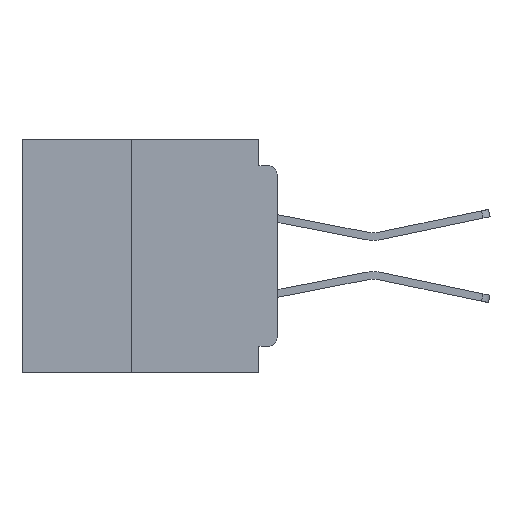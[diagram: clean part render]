
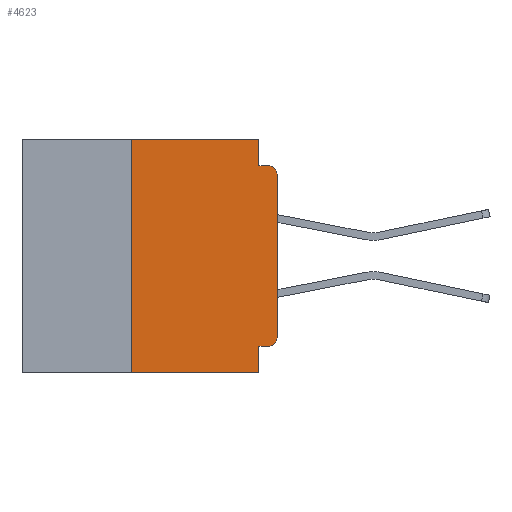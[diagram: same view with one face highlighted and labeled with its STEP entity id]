
A CAD part, left-side view. The second image highlights one B-rep face of the part: STEP entity #4623.
In plain terms, the highlighted planar face has unit normal (-1, 0, 0).
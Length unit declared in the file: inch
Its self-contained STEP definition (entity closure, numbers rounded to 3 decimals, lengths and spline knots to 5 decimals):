
#2740 = AXIS2_PLACEMENT_3D ( 'NONE', #12466, #54005, #53925 ) ;
#3252 = DIRECTION ( 'NONE',  ( 0., -1., 0. ) ) ;
#4163 = EDGE_CURVE ( 'NONE', #45471, #45231, #57447, .T. ) ;
#4395 = LINE ( 'NONE', #33269, #16461 ) ;
#4623 = ADVANCED_FACE ( 'NONE', ( #21454 ), #52763, .F. ) ;
#4956 = DIRECTION ( 'NONE',  ( 0., 0., 1. ) ) ;
#6588 = EDGE_CURVE ( 'NONE', #56029, #7572, #48117, .T. ) ;
#7572 = VERTEX_POINT ( 'NONE', #36489 ) ;
#8348 = DIRECTION ( 'NONE',  ( -1., 0., 0. ) ) ;
#8466 = VERTEX_POINT ( 'NONE', #13797 ) ;
#9559 = ORIENTED_EDGE ( 'NONE', *, *, #12828, .F. ) ;
#11077 = VERTEX_POINT ( 'NONE', #17024 ) ;
#11893 = LINE ( 'NONE', #43286, #58418 ) ;
#12466 = CARTESIAN_POINT ( 'NONE',  ( 0., 0.437, 0. ) ) ;
#12828 = EDGE_CURVE ( 'NONE', #22465, #34806, #11893, .T. ) ;
#13797 = CARTESIAN_POINT ( 'NONE',  ( 0., 0.25, 0. ) ) ;
#14143 = CARTESIAN_POINT ( 'NONE',  ( 0., 0., -0.355 ) ) ;
#14544 = CARTESIAN_POINT ( 'NONE',  ( 0., 0.031, -0.045 ) ) ;
#15021 = ORIENTED_EDGE ( 'NONE', *, *, #6588, .T. ) ;
#15884 = DIRECTION ( 'NONE',  ( -1., 0., 0. ) ) ;
#16260 = DIRECTION ( 'NONE',  ( 0., -1., 0. ) ) ;
#16461 = VECTOR ( 'NONE', #55725, 39.37008 ) ;
#16549 = CARTESIAN_POINT ( 'NONE',  ( 0., 0.015, -0.355 ) ) ;
#16623 = VECTOR ( 'NONE', #16260, 39.37008 ) ;
#17024 = CARTESIAN_POINT ( 'NONE',  ( 0., 0.031, -0.4 ) ) ;
#17712 = EDGE_CURVE ( 'NONE', #42472, #11077, #4395, .T. ) ;
#18859 = ORIENTED_EDGE ( 'NONE', *, *, #36431, .F. ) ;
#21454 = FACE_OUTER_BOUND ( 'NONE', #23707, .T. ) ;
#22059 = EDGE_CURVE ( 'NONE', #34806, #55670, #52582, .T. ) ;
#22465 = VERTEX_POINT ( 'NONE', #33381 ) ;
#23034 = DIRECTION ( 'NONE',  ( 0., 1., 0. ) ) ;
#23264 = ORIENTED_EDGE ( 'NONE', *, *, #17712, .T. ) ;
#23597 = EDGE_CURVE ( 'NONE', #45471, #56029, #47451, .T. ) ;
#23707 = EDGE_LOOP ( 'NONE', ( #15021, #35566, #57545, #9559, #18859, #58197, #23264, #34327, #43718, #28389 ) ) ;
#24941 = DIRECTION ( 'NONE',  ( 0., 0., -1. ) ) ;
#26206 = CARTESIAN_POINT ( 'NONE',  ( 0., 0., -0.34 ) ) ;
#28389 = ORIENTED_EDGE ( 'NONE', *, *, #23597, .T. ) ;
#29040 = LINE ( 'NONE', #47222, #39630 ) ;
#30246 = LINE ( 'NONE', #53013, #40841 ) ;
#32123 = VECTOR ( 'NONE', #23034, 39.37008 ) ;
#32785 = CARTESIAN_POINT ( 'NONE',  ( 0., 0.015, -0.045 ) ) ;
#33144 = CARTESIAN_POINT ( 'NONE',  ( 0., 0.031, -0.355 ) ) ;
#33269 = CARTESIAN_POINT ( 'NONE',  ( 0., 0.437, -0.4 ) ) ;
#33381 = CARTESIAN_POINT ( 'NONE',  ( 0., 0.031, 0. ) ) ;
#34327 = ORIENTED_EDGE ( 'NONE', *, *, #52591, .F. ) ;
#34806 = VERTEX_POINT ( 'NONE', #14544 ) ;
#35189 = EDGE_CURVE ( 'NONE', #7572, #55670, #36740, .T. ) ;
#35338 = EDGE_CURVE ( 'NONE', #42472, #8466, #41681, .T. ) ;
#35416 = CARTESIAN_POINT ( 'NONE',  ( 0., 0.015, -0.06 ) ) ;
#35566 = ORIENTED_EDGE ( 'NONE', *, *, #35189, .T. ) ;
#36387 = CARTESIAN_POINT ( 'NONE',  ( 0., 0.25, -0.4 ) ) ;
#36431 = EDGE_CURVE ( 'NONE', #8466, #22465, #30246, .T. ) ;
#36489 = CARTESIAN_POINT ( 'NONE',  ( 0., 0., -0.06 ) ) ;
#36740 = CIRCLE ( 'NONE', #47551, 0.015 ) ;
#38760 = CARTESIAN_POINT ( 'NONE',  ( 0., 0., 0. ) ) ;
#39630 = VECTOR ( 'NONE', #24941, 39.37008 ) ;
#39955 = DIRECTION ( 'NONE',  ( 0., 0., -1. ) ) ;
#40825 = CARTESIAN_POINT ( 'NONE',  ( 0., 0.25, -0.4 ) ) ;
#40841 = VECTOR ( 'NONE', #3252, 39.37008 ) ;
#41681 = LINE ( 'NONE', #36387, #52216 ) ;
#42472 = VERTEX_POINT ( 'NONE', #40825 ) ;
#42912 = CARTESIAN_POINT ( 'NONE',  ( 0., 0.015, -0.34 ) ) ;
#43286 = CARTESIAN_POINT ( 'NONE',  ( 0., 0.031, 0. ) ) ;
#43483 = DIRECTION ( 'NONE',  ( 0., 0., -1. ) ) ;
#43718 = ORIENTED_EDGE ( 'NONE', *, *, #4163, .F. ) ;
#45231 = VERTEX_POINT ( 'NONE', #33144 ) ;
#45471 = VERTEX_POINT ( 'NONE', #16549 ) ;
#47222 = CARTESIAN_POINT ( 'NONE',  ( 0., 0.031, -0.4 ) ) ;
#47429 = DIRECTION ( 'NONE',  ( 0., 0., -1. ) ) ;
#47451 = CIRCLE ( 'NONE', #57634, 0.015 ) ;
#47551 = AXIS2_PLACEMENT_3D ( 'NONE', #35416, #8348, #39955 ) ;
#48117 = LINE ( 'NONE', #38760, #57229 ) ;
#52216 = VECTOR ( 'NONE', #4956, 39.37008 ) ;
#52308 = CARTESIAN_POINT ( 'NONE',  ( 0., 0., -0.045 ) ) ;
#52582 = LINE ( 'NONE', #52308, #16623 ) ;
#52591 = EDGE_CURVE ( 'NONE', #45231, #11077, #29040, .T. ) ;
#52763 = PLANE ( 'NONE',  #2740 ) ;
#53013 = CARTESIAN_POINT ( 'NONE',  ( 0., 0.437, 0. ) ) ;
#53925 = DIRECTION ( 'NONE',  ( 0., 0., -1. ) ) ;
#54005 = DIRECTION ( 'NONE',  ( 1., 0., 0. ) ) ;
#55670 = VERTEX_POINT ( 'NONE', #32785 ) ;
#55725 = DIRECTION ( 'NONE',  ( 0., -1., 0. ) ) ;
#56029 = VERTEX_POINT ( 'NONE', #26206 ) ;
#56835 = DIRECTION ( 'NONE',  ( 0., 0., 1. ) ) ;
#57229 = VECTOR ( 'NONE', #56835, 39.37008 ) ;
#57447 = LINE ( 'NONE', #14143, #32123 ) ;
#57545 = ORIENTED_EDGE ( 'NONE', *, *, #22059, .F. ) ;
#57634 = AXIS2_PLACEMENT_3D ( 'NONE', #42912, #15884, #47429 ) ;
#58197 = ORIENTED_EDGE ( 'NONE', *, *, #35338, .F. ) ;
#58418 = VECTOR ( 'NONE', #43483, 39.37008 ) ;
